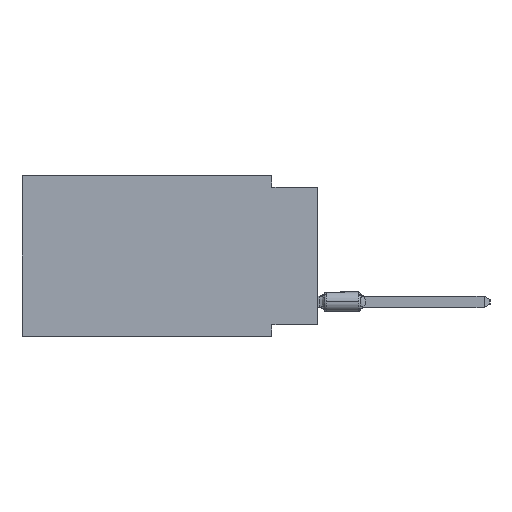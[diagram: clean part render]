
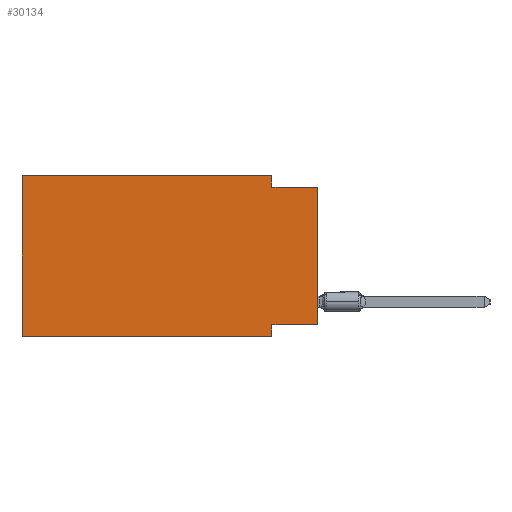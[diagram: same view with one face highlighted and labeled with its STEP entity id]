
A CAD part, left-side view. The second image highlights one B-rep face of the part: STEP entity #30134.
In plain terms, the highlighted planar face has unit normal (-1, 0, 0).
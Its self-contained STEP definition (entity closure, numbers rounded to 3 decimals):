
#1080 = EDGE_LOOP ( 'NONE', ( #4648, #2172, #4334, #27247, #2302, #1131, #16231, #38076 ) ) ;
#1131 = ORIENTED_EDGE ( 'NONE', *, *, #19451, .T. ) ;
#1397 = VERTEX_POINT ( 'NONE', #40494 ) ;
#1524 = DIRECTION ( 'NONE',  ( 0., 0., -1. ) ) ;
#2172 = ORIENTED_EDGE ( 'NONE', *, *, #52401, .F. ) ;
#2302 = ORIENTED_EDGE ( 'NONE', *, *, #28992, .F. ) ;
#4334 = ORIENTED_EDGE ( 'NONE', *, *, #31217, .F. ) ;
#4345 = EDGE_CURVE ( 'NONE', #6323, #53772, #49815, .T. ) ;
#4648 = ORIENTED_EDGE ( 'NONE', *, *, #4345, .T. ) ;
#5010 = VERTEX_POINT ( 'NONE', #24472 ) ;
#6323 = VERTEX_POINT ( 'NONE', #30336 ) ;
#6955 = VECTOR ( 'NONE', #20849, 1000. ) ;
#10741 = VECTOR ( 'NONE', #19102, 1000. ) ;
#11097 = LINE ( 'NONE', #46685, #33582 ) ;
#12374 = CARTESIAN_POINT ( 'NONE',  ( 0., 0., -0.635 ) ) ;
#15027 = FACE_OUTER_BOUND ( 'NONE', #1080, .T. ) ;
#15980 = CARTESIAN_POINT ( 'NONE',  ( 0., 2.54, -8.255 ) ) ;
#16231 = ORIENTED_EDGE ( 'NONE', *, *, #46945, .F. ) ;
#18539 = VECTOR ( 'NONE', #30125, 1000. ) ;
#19102 = DIRECTION ( 'NONE',  ( 0., 0., 1. ) ) ;
#19451 = EDGE_CURVE ( 'NONE', #49200, #25191, #11097, .T. ) ;
#19606 = EDGE_CURVE ( 'NONE', #6323, #36991, #34611, .T. ) ;
#20583 = DIRECTION ( 'NONE',  ( 0., 0., -1. ) ) ;
#20849 = DIRECTION ( 'NONE',  ( 0., 1., 0. ) ) ;
#20855 = VERTEX_POINT ( 'NONE', #44101 ) ;
#23061 = CARTESIAN_POINT ( 'NONE',  ( 0., 16.383, 0. ) ) ;
#23356 = CARTESIAN_POINT ( 'NONE',  ( 0., 16.383, 0. ) ) ;
#24472 = CARTESIAN_POINT ( 'NONE',  ( 0., 16.383, 0. ) ) ;
#25191 = VERTEX_POINT ( 'NONE', #40826 ) ;
#27247 = ORIENTED_EDGE ( 'NONE', *, *, #41717, .F. ) ;
#28887 = DIRECTION ( 'NONE',  ( 0., -1., 0. ) ) ;
#28992 = EDGE_CURVE ( 'NONE', #49200, #5010, #51951, .T. ) ;
#29188 = LINE ( 'NONE', #46703, #55928 ) ;
#29876 = LINE ( 'NONE', #12374, #54647 ) ;
#30125 = DIRECTION ( 'NONE',  ( 0., 0., 1. ) ) ;
#30134 = ADVANCED_FACE ( 'NONE', ( #15027 ), #44883, .F. ) ;
#30336 = CARTESIAN_POINT ( 'NONE',  ( 0., 0., -8.255 ) ) ;
#31217 = EDGE_CURVE ( 'NONE', #20855, #1397, #29188, .T. ) ;
#31473 = CARTESIAN_POINT ( 'NONE',  ( 0., 0., 0. ) ) ;
#31582 = DIRECTION ( 'NONE',  ( 0., 0., -1. ) ) ;
#31683 = DIRECTION ( 'NONE',  ( 1., 0., 0. ) ) ;
#31853 = CARTESIAN_POINT ( 'NONE',  ( 0., 2.54, -8.89 ) ) ;
#31990 = AXIS2_PLACEMENT_3D ( 'NONE', #23356, #31683, #1524 ) ;
#33582 = VECTOR ( 'NONE', #28887, 1000. ) ;
#33898 = DIRECTION ( 'NONE',  ( 0., -1., 0. ) ) ;
#34611 = LINE ( 'NONE', #38650, #6955 ) ;
#36991 = VERTEX_POINT ( 'NONE', #15980 ) ;
#38076 = ORIENTED_EDGE ( 'NONE', *, *, #19606, .F. ) ;
#38650 = CARTESIAN_POINT ( 'NONE',  ( 0., 0., -8.255 ) ) ;
#39347 = CARTESIAN_POINT ( 'NONE',  ( 0., 16.383, -8.89 ) ) ;
#40494 = CARTESIAN_POINT ( 'NONE',  ( 0., 2.54, -0.635 ) ) ;
#40826 = CARTESIAN_POINT ( 'NONE',  ( 0., 2.54, -8.89 ) ) ;
#41500 = VECTOR ( 'NONE', #53212, 1000. ) ;
#41717 = EDGE_CURVE ( 'NONE', #5010, #20855, #44579, .T. ) ;
#44101 = CARTESIAN_POINT ( 'NONE',  ( 0., 2.54, 0. ) ) ;
#44579 = LINE ( 'NONE', #23061, #41500 ) ;
#44883 = PLANE ( 'NONE',  #31990 ) ;
#46685 = CARTESIAN_POINT ( 'NONE',  ( 0., 16.383, -8.89 ) ) ;
#46703 = CARTESIAN_POINT ( 'NONE',  ( 0., 2.54, 0. ) ) ;
#46945 = EDGE_CURVE ( 'NONE', #36991, #25191, #48811, .T. ) ;
#47021 = VECTOR ( 'NONE', #31582, 1000. ) ;
#48201 = CARTESIAN_POINT ( 'NONE',  ( 0., 16.383, 0. ) ) ;
#48811 = LINE ( 'NONE', #31853, #47021 ) ;
#49200 = VERTEX_POINT ( 'NONE', #39347 ) ;
#49815 = LINE ( 'NONE', #31473, #10741 ) ;
#51951 = LINE ( 'NONE', #48201, #18539 ) ;
#52401 = EDGE_CURVE ( 'NONE', #1397, #53772, #29876, .T. ) ;
#53212 = DIRECTION ( 'NONE',  ( 0., -1., 0. ) ) ;
#53772 = VERTEX_POINT ( 'NONE', #54721 ) ;
#54647 = VECTOR ( 'NONE', #33898, 1000. ) ;
#54721 = CARTESIAN_POINT ( 'NONE',  ( 0., 0., -0.635 ) ) ;
#55928 = VECTOR ( 'NONE', #20583, 1000. ) ;
